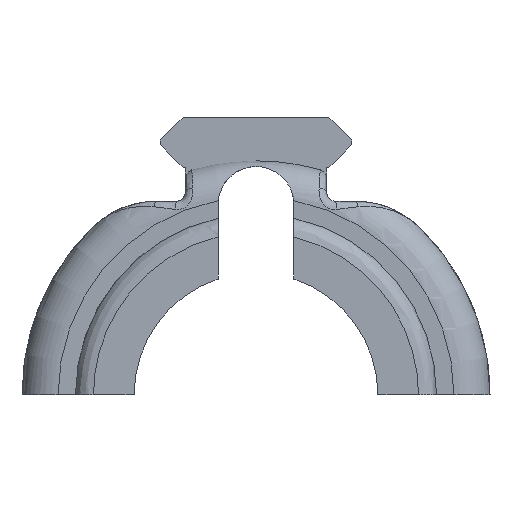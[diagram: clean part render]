
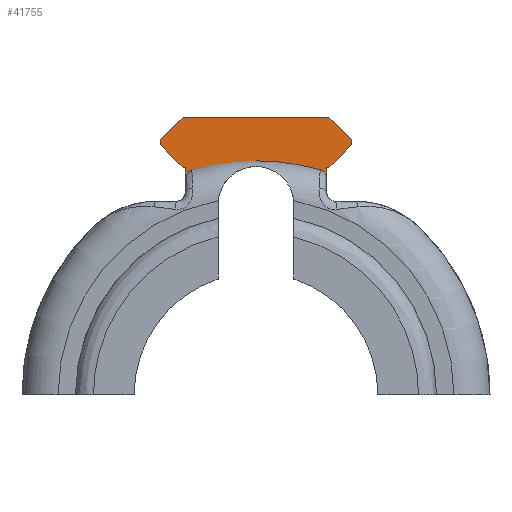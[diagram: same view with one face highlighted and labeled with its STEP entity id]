
A CAD part, left-side view. The second image highlights one B-rep face of the part: STEP entity #41755.
In plain terms, the highlighted planar face has unit normal (-1, 0, 0).
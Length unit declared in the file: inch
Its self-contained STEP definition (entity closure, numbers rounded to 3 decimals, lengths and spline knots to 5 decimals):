
#55 = ORIENTED_EDGE ( 'NONE', *, *, #33469, .T. ) ;
#64 = CARTESIAN_POINT ( 'NONE',  ( 0., 0.32901, 0.9435 ) ) ;
#2705 = DIRECTION ( 'NONE',  ( 0., -1., 0. ) ) ;
#3034 = ORIENTED_EDGE ( 'NONE', *, *, #57371, .T. ) ;
#4102 = ORIENTED_EDGE ( 'NONE', *, *, #4437, .T. ) ;
#4437 = EDGE_CURVE ( 'NONE', #64836, #61117, #86021, .T. ) ;
#4729 = CARTESIAN_POINT ( 'NONE',  ( 0., 0.02051, 0. ) ) ;
#4820 = ORIENTED_EDGE ( 'NONE', *, *, #81772, .T. ) ;
#6002 = VECTOR ( 'NONE', #50656, 39.37008 ) ;
#6197 = EDGE_CURVE ( 'NONE', #46208, #84711, #82329, .T. ) ;
#6766 = ORIENTED_EDGE ( 'NONE', *, *, #56678, .T. ) ;
#6852 = EDGE_CURVE ( 'NONE', #37856, #12527, #24914, .T. ) ;
#7603 = LINE ( 'NONE', #81931, #24474 ) ;
#8949 = DIRECTION ( 'NONE',  ( 0., 1., 0. ) ) ;
#9448 = CARTESIAN_POINT ( 'NONE',  ( 0., 0.30044, 0.98136 ) ) ;
#9616 = ORIENTED_EDGE ( 'NONE', *, *, #46494, .T. ) ;
#9931 = CARTESIAN_POINT ( 'NONE',  ( 0., -0.39699, 1.1115 ) ) ;
#10809 = VECTOR ( 'NONE', #90002, 39.37008 ) ;
#10836 = EDGE_CURVE ( 'NONE', #61117, #37856, #7603, .T. ) ;
#11071 = CARTESIAN_POINT ( 'NONE',  ( 0., 0.33851, 1.211 ) ) ;
#11963 = DIRECTION ( 'NONE',  ( 0., -1., 0. ) ) ;
#12246 = CARTESIAN_POINT ( 'NONE',  ( 0., 0.39451, 1.155 ) ) ;
#12397 = CARTESIAN_POINT ( 'NONE',  ( 0., -0.28799, 0.991 ) ) ;
#12527 = VERTEX_POINT ( 'NONE', #9448 ) ;
#12633 = EDGE_CURVE ( 'NONE', #84711, #33863, #58845, .T. ) ;
#12717 = VECTOR ( 'NONE', #35962, 39.37008 ) ;
#13588 = DIRECTION ( 'NONE',  ( 0., -1., 0. ) ) ;
#13617 = CARTESIAN_POINT ( 'NONE',  ( 0., 0.32901, 0.991 ) ) ;
#14606 = VECTOR ( 'NONE', #68820, 39.37008 ) ;
#15218 = CARTESIAN_POINT ( 'NONE',  ( 0., 0.33851, 0.991 ) ) ;
#15724 = DIRECTION ( 'NONE',  ( -1., 0., 0. ) ) ;
#15732 = DIRECTION ( 'NONE',  ( 1., 0., 0. ) ) ;
#15736 = LINE ( 'NONE', #70363, #17988 ) ;
#16205 = CARTESIAN_POINT ( 'NONE',  ( 0., 0.33851, 1.211 ) ) ;
#17009 = CARTESIAN_POINT ( 'NONE',  ( 0., -0.39699, 1.0905 ) ) ;
#17988 = VECTOR ( 'NONE', #19072, 39.37008 ) ;
#18646 = VERTEX_POINT ( 'NONE', #23693 ) ;
#19072 = DIRECTION ( 'NONE',  ( 0., 0.707, 0.707 ) ) ;
#19499 = ORIENTED_EDGE ( 'NONE', *, *, #24434, .F. ) ;
#21141 = CARTESIAN_POINT ( 'NONE',  ( 0., -0.39699, 1.1115 ) ) ;
#21465 = VERTEX_POINT ( 'NONE', #32166 ) ;
#22688 = AXIS2_PLACEMENT_3D ( 'NONE', #58257, #15732, #65273 ) ;
#23693 = CARTESIAN_POINT ( 'NONE',  ( 0., 0.43801, 1.0905 ) ) ;
#24434 = EDGE_CURVE ( 'NONE', #76720, #33990, #34587, .T. ) ;
#24474 = VECTOR ( 'NONE', #53777, 39.37008 ) ;
#24700 = AXIS2_PLACEMENT_3D ( 'NONE', #87478, #45382, #2705 ) ;
#24914 = CIRCLE ( 'NONE', #22688, 0.03937 ) ;
#27071 = VERTEX_POINT ( 'NONE', #17009 ) ;
#29556 = AXIS2_PLACEMENT_3D ( 'NONE', #58252, #15724, #65265 ) ;
#32166 = CARTESIAN_POINT ( 'NONE',  ( 0., -0.28799, 0.9435 ) ) ;
#32557 = ORIENTED_EDGE ( 'NONE', *, *, #65869, .T. ) ;
#33469 = EDGE_CURVE ( 'NONE', #47839, #46208, #15736, .T. ) ;
#33863 = VERTEX_POINT ( 'NONE', #37517 ) ;
#33990 = VERTEX_POINT ( 'NONE', #46773 ) ;
#34196 = VECTOR ( 'NONE', #43232, 39.37008 ) ;
#34587 = CIRCLE ( 'NONE', #29556, 1.02051 ) ;
#34761 = CARTESIAN_POINT ( 'NONE',  ( 0., 0.02051, 1.529 ) ) ;
#35907 = VECTOR ( 'NONE', #91494, 39.37008 ) ;
#35962 = DIRECTION ( 'NONE',  ( 0., -0.707, 0.707 ) ) ;
#37517 = CARTESIAN_POINT ( 'NONE',  ( 0., 0.43801, 1.1115 ) ) ;
#37856 = VERTEX_POINT ( 'NONE', #64 ) ;
#38934 = ORIENTED_EDGE ( 'NONE', *, *, #6852, .T. ) ;
#39322 = EDGE_CURVE ( 'NONE', #33990, #12527, #48900, .T. ) ;
#40948 = FACE_OUTER_BOUND ( 'NONE', #69104, .T. ) ;
#41755 = ADVANCED_FACE ( 'NONE', ( #40948 ), #49027, .T. ) ;
#43161 = DIRECTION ( 'NONE',  ( 0., 0., 1. ) ) ;
#43232 = DIRECTION ( 'NONE',  ( 0., 0., -1. ) ) ;
#45382 = DIRECTION ( 'NONE',  ( 1., 0., 0. ) ) ;
#46208 = VERTEX_POINT ( 'NONE', #91439 ) ;
#46494 = EDGE_CURVE ( 'NONE', #33863, #18646, #53127, .T. ) ;
#46773 = CARTESIAN_POINT ( 'NONE',  ( 0., 0.02051, 1.02051 ) ) ;
#47618 = AXIS2_PLACEMENT_3D ( 'NONE', #34761, #56169, #13588 ) ;
#47839 = VERTEX_POINT ( 'NONE', #9931 ) ;
#48301 = LINE ( 'NONE', #78205, #12717 ) ;
#48609 = CIRCLE ( 'NONE', #24700, 0.03937 ) ;
#48900 = CIRCLE ( 'NONE', #62374, 1.02051 ) ;
#49027 = PLANE ( 'NONE',  #47618 ) ;
#49317 = CARTESIAN_POINT ( 'NONE',  ( 0., -0.25942, 0.98136 ) ) ;
#49807 = CARTESIAN_POINT ( 'NONE',  ( 0., 0.43801, 1.1115 ) ) ;
#50656 = DIRECTION ( 'NONE',  ( 0., -1., 0. ) ) ;
#52167 = ORIENTED_EDGE ( 'NONE', *, *, #10836, .T. ) ;
#53127 = LINE ( 'NONE', #49807, #34196 ) ;
#53777 = DIRECTION ( 'NONE',  ( 0., 0., -1. ) ) ;
#54599 = DIRECTION ( 'NONE',  ( -1., 0., 0. ) ) ;
#54805 = ORIENTED_EDGE ( 'NONE', *, *, #65225, .T. ) ;
#56169 = DIRECTION ( 'NONE',  ( -1., 0., 0. ) ) ;
#56678 = EDGE_CURVE ( 'NONE', #27071, #47839, #84298, .T. ) ;
#57371 = EDGE_CURVE ( 'NONE', #18646, #64836, #75675, .T. ) ;
#58252 = CARTESIAN_POINT ( 'NONE',  ( 0., 0.02051, 0. ) ) ;
#58257 = CARTESIAN_POINT ( 'NONE',  ( 0., 0.28964, 0.9435 ) ) ;
#58397 = LINE ( 'NONE', #71535, #6002 ) ;
#58845 = LINE ( 'NONE', #12246, #77448 ) ;
#58999 = EDGE_CURVE ( 'NONE', #21465, #62415, #66728, .T. ) ;
#61117 = VERTEX_POINT ( 'NONE', #13617 ) ;
#62374 = AXIS2_PLACEMENT_3D ( 'NONE', #4729, #54599, #11963 ) ;
#62415 = VERTEX_POINT ( 'NONE', #87587 ) ;
#63686 = VECTOR ( 'NONE', #8949, 39.37008 ) ;
#64836 = VERTEX_POINT ( 'NONE', #85976 ) ;
#64881 = ORIENTED_EDGE ( 'NONE', *, *, #12633, .T. ) ;
#65225 = EDGE_CURVE ( 'NONE', #62415, #88034, #58397, .T. ) ;
#65265 = DIRECTION ( 'NONE',  ( 0., -1., 0. ) ) ;
#65273 = DIRECTION ( 'NONE',  ( 0., -1., 0. ) ) ;
#65720 = VECTOR ( 'NONE', #43161, 39.37008 ) ;
#65869 = EDGE_CURVE ( 'NONE', #88034, #27071, #48301, .T. ) ;
#66728 = LINE ( 'NONE', #12397, #14606 ) ;
#68820 = DIRECTION ( 'NONE',  ( 0., 0., 1. ) ) ;
#68972 = DIRECTION ( 'NONE',  ( 0., 0.707, -0.707 ) ) ;
#69104 = EDGE_LOOP ( 'NONE', ( #19499, #4820, #84389, #54805, #32557, #6766, #55, #84409, #64881, #9616, #3034, #4102, #52167, #38934, #69942 ) ) ;
#69571 = CARTESIAN_POINT ( 'NONE',  ( 0., 0.39451, 1.047 ) ) ;
#69942 = ORIENTED_EDGE ( 'NONE', *, *, #39322, .F. ) ;
#70363 = CARTESIAN_POINT ( 'NONE',  ( 0., -0.35349, 1.155 ) ) ;
#71535 = CARTESIAN_POINT ( 'NONE',  ( 0., -0.28799, 0.991 ) ) ;
#75675 = LINE ( 'NONE', #69571, #35907 ) ;
#75981 = CARTESIAN_POINT ( 'NONE',  ( 0., -0.29749, 0.991 ) ) ;
#76720 = VERTEX_POINT ( 'NONE', #49317 ) ;
#77448 = VECTOR ( 'NONE', #68972, 39.37008 ) ;
#78205 = CARTESIAN_POINT ( 'NONE',  ( 0., -0.39699, 1.0905 ) ) ;
#81772 = EDGE_CURVE ( 'NONE', #76720, #21465, #48609, .T. ) ;
#81931 = CARTESIAN_POINT ( 'NONE',  ( 0., 0.32901, 0.991 ) ) ;
#82329 = LINE ( 'NONE', #16205, #63686 ) ;
#84298 = LINE ( 'NONE', #21141, #65720 ) ;
#84389 = ORIENTED_EDGE ( 'NONE', *, *, #58999, .T. ) ;
#84409 = ORIENTED_EDGE ( 'NONE', *, *, #6197, .T. ) ;
#84711 = VERTEX_POINT ( 'NONE', #11071 ) ;
#85976 = CARTESIAN_POINT ( 'NONE',  ( 0., 0.33851, 0.991 ) ) ;
#86021 = LINE ( 'NONE', #15218, #10809 ) ;
#87478 = CARTESIAN_POINT ( 'NONE',  ( 0., -0.24862, 0.9435 ) ) ;
#87587 = CARTESIAN_POINT ( 'NONE',  ( 0., -0.28799, 0.991 ) ) ;
#88034 = VERTEX_POINT ( 'NONE', #75981 ) ;
#90002 = DIRECTION ( 'NONE',  ( 0., -1., 0. ) ) ;
#91439 = CARTESIAN_POINT ( 'NONE',  ( 0., -0.29749, 1.211 ) ) ;
#91494 = DIRECTION ( 'NONE',  ( 0., -0.707, -0.707 ) ) ;
